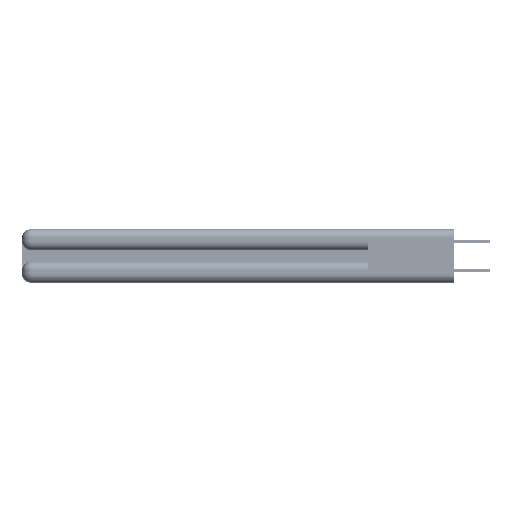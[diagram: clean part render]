
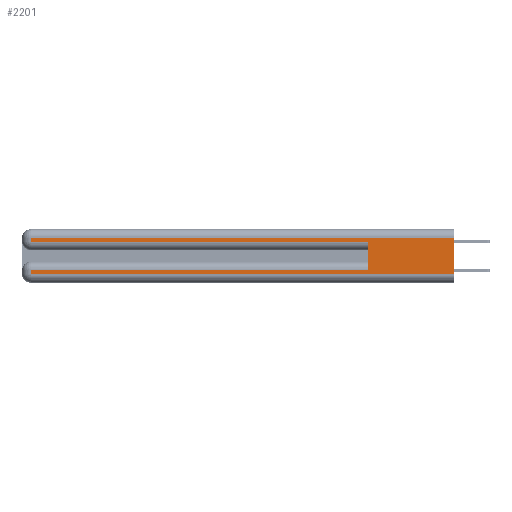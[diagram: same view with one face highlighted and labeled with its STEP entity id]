
A CAD part, left-side view. The second image highlights one B-rep face of the part: STEP entity #2201.
In plain terms, the highlighted planar face has unit normal (-1, 0, 0).
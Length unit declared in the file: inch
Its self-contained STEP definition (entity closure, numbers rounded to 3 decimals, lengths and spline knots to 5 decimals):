
#937 = EDGE_CURVE ( 'NONE', #28319, #35123, #20153, .T. ) ;
#2201 = ADVANCED_FACE ( 'NONE', ( #16234 ), #23624, .F. ) ;
#2542 = CARTESIAN_POINT ( 'NONE',  ( 0., 0., 0.37 ) ) ;
#3193 = CARTESIAN_POINT ( 'NONE',  ( 0., 2.94, 0.37 ) ) ;
#3502 = CARTESIAN_POINT ( 'NONE',  ( 0., 2.94, 0.31 ) ) ;
#3526 = EDGE_LOOP ( 'NONE', ( #3550, #14334, #15993, #15525, #27177, #19827, #40036, #39657 ) ) ;
#3550 = ORIENTED_EDGE ( 'NONE', *, *, #12709, .F. ) ;
#5184 = VERTEX_POINT ( 'NONE', #41917 ) ;
#5399 = VECTOR ( 'NONE', #13060, 39.37008 ) ;
#6115 = CARTESIAN_POINT ( 'NONE',  ( 0., 2.94, 0.085 ) ) ;
#6945 = VERTEX_POINT ( 'NONE', #18758 ) ;
#7843 = VECTOR ( 'NONE', #15409, 39.37008 ) ;
#7937 = EDGE_CURVE ( 'NONE', #9618, #6945, #40561, .T. ) ;
#8138 = DIRECTION ( 'NONE',  ( 0., -1., 0. ) ) ;
#8876 = VECTOR ( 'NONE', #8138, 39.37008 ) ;
#9618 = VERTEX_POINT ( 'NONE', #30516 ) ;
#12709 = EDGE_CURVE ( 'NONE', #22661, #5184, #16312, .T. ) ;
#13060 = DIRECTION ( 'NONE',  ( 0., 0., -1. ) ) ;
#14105 = DIRECTION ( 'NONE',  ( 0., 0., -1. ) ) ;
#14334 = ORIENTED_EDGE ( 'NONE', *, *, #29501, .T. ) ;
#14904 = LINE ( 'NONE', #32668, #36383 ) ;
#15409 = DIRECTION ( 'NONE',  ( 0., 1., 0. ) ) ;
#15525 = ORIENTED_EDGE ( 'NONE', *, *, #39732, .T. ) ;
#15993 = ORIENTED_EDGE ( 'NONE', *, *, #937, .T. ) ;
#16234 = FACE_OUTER_BOUND ( 'NONE', #3526, .T. ) ;
#16312 = LINE ( 'NONE', #2542, #41973 ) ;
#18758 = CARTESIAN_POINT ( 'NONE',  ( 0., 0.6, 0.285 ) ) ;
#18991 = CARTESIAN_POINT ( 'NONE',  ( 0., 0.6, 0.145 ) ) ;
#19827 = ORIENTED_EDGE ( 'NONE', *, *, #25510, .T. ) ;
#20153 = LINE ( 'NONE', #30495, #24266 ) ;
#20733 = VERTEX_POINT ( 'NONE', #6115 ) ;
#20843 = LINE ( 'NONE', #34981, #8876 ) ;
#21845 = LINE ( 'NONE', #40598, #38551 ) ;
#21973 = LINE ( 'NONE', #39096, #7843 ) ;
#22661 = VERTEX_POINT ( 'NONE', #42755 ) ;
#23358 = VECTOR ( 'NONE', #25548, 39.37008 ) ;
#23624 = PLANE ( 'NONE',  #37411 ) ;
#24266 = VECTOR ( 'NONE', #37881, 39.37008 ) ;
#25510 = EDGE_CURVE ( 'NONE', #9618, #20733, #14904, .T. ) ;
#25548 = DIRECTION ( 'NONE',  ( 0., 0., 1. ) ) ;
#26450 = CARTESIAN_POINT ( 'NONE',  ( 0., 0., 0.37 ) ) ;
#27177 = ORIENTED_EDGE ( 'NONE', *, *, #7937, .F. ) ;
#27185 = DIRECTION ( 'NONE',  ( 0., -1., 0. ) ) ;
#28319 = VERTEX_POINT ( 'NONE', #3502 ) ;
#29501 = EDGE_CURVE ( 'NONE', #22661, #28319, #21973, .T. ) ;
#30279 = CARTESIAN_POINT ( 'NONE',  ( 0., 2.94, 0.06 ) ) ;
#30495 = CARTESIAN_POINT ( 'NONE',  ( 0., 2.94, 0.37 ) ) ;
#30516 = CARTESIAN_POINT ( 'NONE',  ( 0., 0.6, 0.085 ) ) ;
#32287 = VERTEX_POINT ( 'NONE', #30279 ) ;
#32668 = CARTESIAN_POINT ( 'NONE',  ( 0., 0., 0.085 ) ) ;
#32813 = DIRECTION ( 'NONE',  ( 0., 1., 0. ) ) ;
#34349 = EDGE_CURVE ( 'NONE', #20733, #32287, #41987, .T. ) ;
#34981 = CARTESIAN_POINT ( 'NONE',  ( 0., 0., 0.06 ) ) ;
#35123 = VERTEX_POINT ( 'NONE', #41239 ) ;
#36383 = VECTOR ( 'NONE', #32813, 39.37008 ) ;
#36451 = EDGE_CURVE ( 'NONE', #32287, #5184, #20843, .T. ) ;
#37411 = AXIS2_PLACEMENT_3D ( 'NONE', #26450, #39885, #40414 ) ;
#37881 = DIRECTION ( 'NONE',  ( 0., 0., -1. ) ) ;
#38551 = VECTOR ( 'NONE', #27185, 39.37008 ) ;
#39096 = CARTESIAN_POINT ( 'NONE',  ( 0., 0., 0.31 ) ) ;
#39657 = ORIENTED_EDGE ( 'NONE', *, *, #36451, .T. ) ;
#39732 = EDGE_CURVE ( 'NONE', #35123, #6945, #21845, .T. ) ;
#39885 = DIRECTION ( 'NONE',  ( 1., 0., 0. ) ) ;
#40036 = ORIENTED_EDGE ( 'NONE', *, *, #34349, .T. ) ;
#40414 = DIRECTION ( 'NONE',  ( 0., 0., -1. ) ) ;
#40561 = LINE ( 'NONE', #18991, #23358 ) ;
#40598 = CARTESIAN_POINT ( 'NONE',  ( 0., 0., 0.285 ) ) ;
#41239 = CARTESIAN_POINT ( 'NONE',  ( 0., 2.94, 0.285 ) ) ;
#41917 = CARTESIAN_POINT ( 'NONE',  ( 0., 0., 0.06 ) ) ;
#41973 = VECTOR ( 'NONE', #14105, 39.37008 ) ;
#41987 = LINE ( 'NONE', #3193, #5399 ) ;
#42755 = CARTESIAN_POINT ( 'NONE',  ( 0., 0., 0.31 ) ) ;
